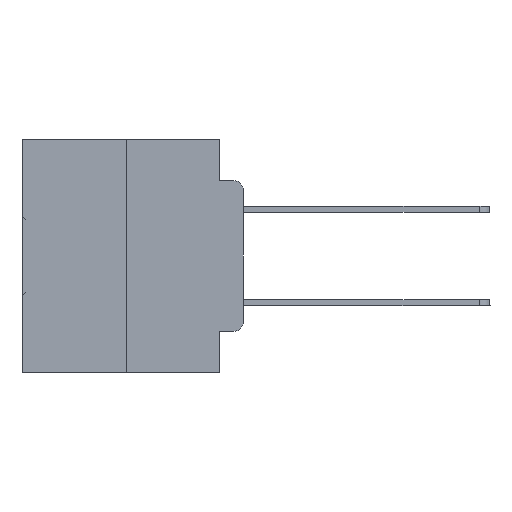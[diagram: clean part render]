
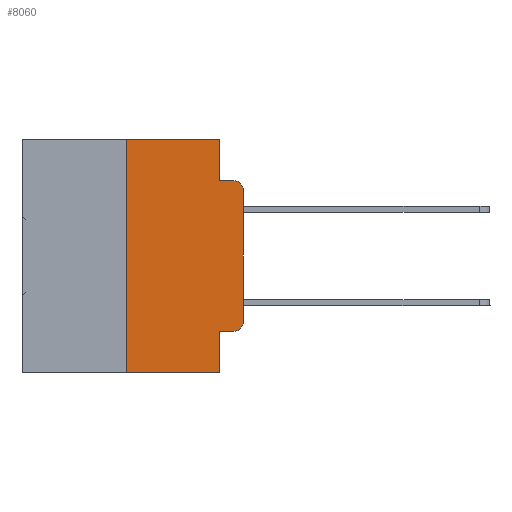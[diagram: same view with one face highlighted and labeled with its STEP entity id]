
A CAD part, left-side view. The second image highlights one B-rep face of the part: STEP entity #8060.
In plain terms, the highlighted planar face has unit normal (-1, 0, 0).
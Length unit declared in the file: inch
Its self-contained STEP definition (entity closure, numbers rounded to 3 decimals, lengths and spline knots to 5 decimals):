
#980 = VERTEX_POINT ( 'NONE', #30706 ) ;
#1098 = CARTESIAN_POINT ( 'NONE',  ( 0., 0.473, 0. ) ) ;
#1200 = FACE_OUTER_BOUND ( 'NONE', #34145, .T. ) ;
#1223 = DIRECTION ( 'NONE',  ( -1., 0., 0. ) ) ;
#1566 = CARTESIAN_POINT ( 'NONE',  ( 0., 0.473, 0. ) ) ;
#1894 = LINE ( 'NONE', #20897, #16955 ) ;
#2118 = ORIENTED_EDGE ( 'NONE', *, *, #8193, .F. ) ;
#2129 = CARTESIAN_POINT ( 'NONE',  ( 0., 0.473, -0.5 ) ) ;
#2163 = DIRECTION ( 'NONE',  ( 0., 0., -1. ) ) ;
#2377 = DIRECTION ( 'NONE',  ( 0., 0., -1. ) ) ;
#2750 = CARTESIAN_POINT ( 'NONE',  ( 0., 0.051, -0.5 ) ) ;
#4216 = PLANE ( 'NONE',  #19957 ) ;
#4797 = LINE ( 'NONE', #29270, #7549 ) ;
#5055 = LINE ( 'NONE', #10375, #32910 ) ;
#5309 = AXIS2_PLACEMENT_3D ( 'NONE', #31371, #18266, #23375 ) ;
#5341 = LINE ( 'NONE', #10692, #17954 ) ;
#5550 = VERTEX_POINT ( 'NONE', #32336 ) ;
#6189 = EDGE_CURVE ( 'NONE', #11878, #22241, #1894, .T. ) ;
#6292 = ORIENTED_EDGE ( 'NONE', *, *, #31066, .T. ) ;
#6840 = EDGE_CURVE ( 'NONE', #31974, #16802, #5055, .T. ) ;
#6909 = DIRECTION ( 'NONE',  ( 0., 0., -1. ) ) ;
#7054 = DIRECTION ( 'NONE',  ( 0., -1., 0. ) ) ;
#7255 = EDGE_CURVE ( 'NONE', #14036, #11878, #5341, .T. ) ;
#7299 = DIRECTION ( 'NONE',  ( 0., -1., 0. ) ) ;
#7549 = VECTOR ( 'NONE', #7299, 39.37008 ) ;
#8060 = ADVANCED_FACE ( 'NONE', ( #1200 ), #4216, .F. ) ;
#8193 = EDGE_CURVE ( 'NONE', #980, #33365, #34655, .T. ) ;
#8701 = CIRCLE ( 'NONE', #5309, 0.02 ) ;
#8760 = DIRECTION ( 'NONE',  ( 0., 0., 1. ) ) ;
#10091 = AXIS2_PLACEMENT_3D ( 'NONE', #19876, #1223, #6909 ) ;
#10336 = CARTESIAN_POINT ( 'NONE',  ( 0., 0.051, -0.0885 ) ) ;
#10375 = CARTESIAN_POINT ( 'NONE',  ( 0., 0.051, 0. ) ) ;
#10692 = CARTESIAN_POINT ( 'NONE',  ( 0., 0.051, 0. ) ) ;
#11146 = VECTOR ( 'NONE', #25566, 39.37008 ) ;
#11205 = CARTESIAN_POINT ( 'NONE',  ( 0., 0., 0. ) ) ;
#11878 = VERTEX_POINT ( 'NONE', #10336 ) ;
#12017 = ORIENTED_EDGE ( 'NONE', *, *, #14359, .F. ) ;
#12404 = DIRECTION ( 'NONE',  ( 1., 0., 0. ) ) ;
#12962 = LINE ( 'NONE', #2129, #19179 ) ;
#13619 = VERTEX_POINT ( 'NONE', #28567 ) ;
#13621 = ORIENTED_EDGE ( 'NONE', *, *, #6189, .F. ) ;
#14036 = VERTEX_POINT ( 'NONE', #33417 ) ;
#14359 = EDGE_CURVE ( 'NONE', #33365, #14036, #28592, .T. ) ;
#14846 = CARTESIAN_POINT ( 'NONE',  ( 0., 0.02, -0.0885 ) ) ;
#16518 = VERTEX_POINT ( 'NONE', #28156 ) ;
#16721 = ORIENTED_EDGE ( 'NONE', *, *, #23740, .T. ) ;
#16802 = VERTEX_POINT ( 'NONE', #2750 ) ;
#16955 = VECTOR ( 'NONE', #7054, 39.37008 ) ;
#17708 = EDGE_CURVE ( 'NONE', #980, #16802, #12962, .T. ) ;
#17755 = ORIENTED_EDGE ( 'NONE', *, *, #6840, .F. ) ;
#17850 = CARTESIAN_POINT ( 'NONE',  ( 0., 0.25, 0. ) ) ;
#17954 = VECTOR ( 'NONE', #2163, 39.37008 ) ;
#18136 = DIRECTION ( 'NONE',  ( 0., -1., 0. ) ) ;
#18266 = DIRECTION ( 'NONE',  ( -1., 0., 0. ) ) ;
#19179 = VECTOR ( 'NONE', #18136, 39.37008 ) ;
#19876 = CARTESIAN_POINT ( 'NONE',  ( 0., 0.02, -0.3915 ) ) ;
#19957 = AXIS2_PLACEMENT_3D ( 'NONE', #1566, #12404, #23209 ) ;
#20872 = CIRCLE ( 'NONE', #10091, 0.02 ) ;
#20897 = CARTESIAN_POINT ( 'NONE',  ( 0., 0.051, -0.0885 ) ) ;
#22241 = VERTEX_POINT ( 'NONE', #14846 ) ;
#22263 = CARTESIAN_POINT ( 'NONE',  ( 0., 0.051, -0.4115 ) ) ;
#23209 = DIRECTION ( 'NONE',  ( 0., 0., -1. ) ) ;
#23210 = ORIENTED_EDGE ( 'NONE', *, *, #7255, .F. ) ;
#23375 = DIRECTION ( 'NONE',  ( 0., 0., -1. ) ) ;
#23740 = EDGE_CURVE ( 'NONE', #5550, #22241, #8701, .T. ) ;
#24727 = EDGE_CURVE ( 'NONE', #31974, #16518, #4797, .T. ) ;
#25566 = DIRECTION ( 'NONE',  ( 0., -1., 0. ) ) ;
#26015 = ORIENTED_EDGE ( 'NONE', *, *, #17708, .T. ) ;
#27848 = DIRECTION ( 'NONE',  ( 0., 0., 1. ) ) ;
#28019 = LINE ( 'NONE', #11205, #29759 ) ;
#28156 = CARTESIAN_POINT ( 'NONE',  ( 0., 0.02, -0.4115 ) ) ;
#28567 = CARTESIAN_POINT ( 'NONE',  ( 0., 0., -0.3915 ) ) ;
#28592 = LINE ( 'NONE', #1098, #11146 ) ;
#29270 = CARTESIAN_POINT ( 'NONE',  ( 0., 0.051, -0.4115 ) ) ;
#29759 = VECTOR ( 'NONE', #27848, 39.37008 ) ;
#30108 = ORIENTED_EDGE ( 'NONE', *, *, #34176, .T. ) ;
#30706 = CARTESIAN_POINT ( 'NONE',  ( 0., 0.25, -0.5 ) ) ;
#31066 = EDGE_CURVE ( 'NONE', #16518, #13619, #20872, .T. ) ;
#31371 = CARTESIAN_POINT ( 'NONE',  ( 0., 0.02, -0.1085 ) ) ;
#31974 = VERTEX_POINT ( 'NONE', #22263 ) ;
#32006 = CARTESIAN_POINT ( 'NONE',  ( 0., 0.25, 0. ) ) ;
#32336 = CARTESIAN_POINT ( 'NONE',  ( 0., 0., -0.1085 ) ) ;
#32910 = VECTOR ( 'NONE', #2377, 39.37008 ) ;
#32945 = VECTOR ( 'NONE', #8760, 39.37008 ) ;
#33365 = VERTEX_POINT ( 'NONE', #17850 ) ;
#33417 = CARTESIAN_POINT ( 'NONE',  ( 0., 0.051, 0. ) ) ;
#34145 = EDGE_LOOP ( 'NONE', ( #30108, #16721, #13621, #23210, #12017, #2118, #26015, #17755, #34534, #6292 ) ) ;
#34176 = EDGE_CURVE ( 'NONE', #13619, #5550, #28019, .T. ) ;
#34534 = ORIENTED_EDGE ( 'NONE', *, *, #24727, .T. ) ;
#34655 = LINE ( 'NONE', #32006, #32945 ) ;
